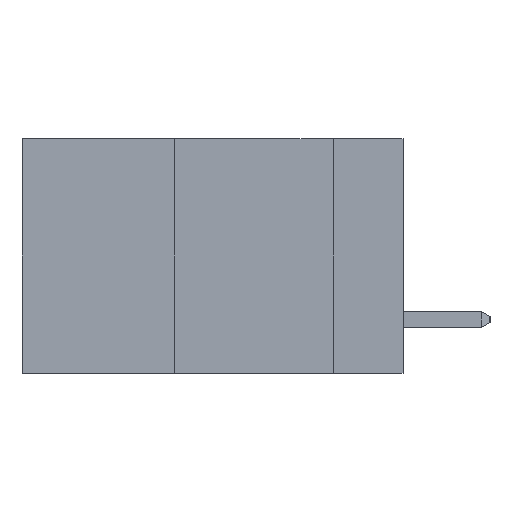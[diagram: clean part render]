
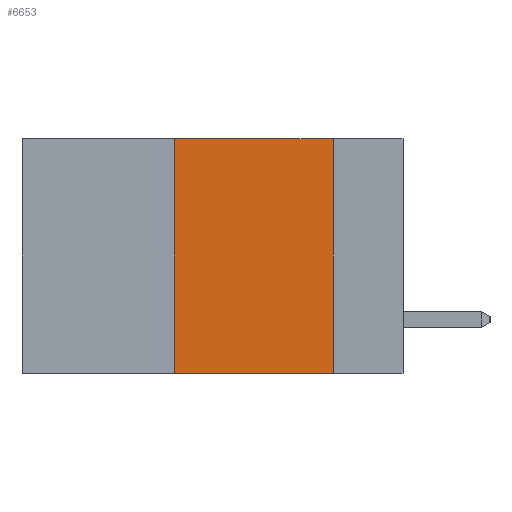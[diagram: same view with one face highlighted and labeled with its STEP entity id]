
A CAD part, left-side view. The second image highlights one B-rep face of the part: STEP entity #6653.
In plain terms, the highlighted planar face has unit normal (-1, 0, 0).
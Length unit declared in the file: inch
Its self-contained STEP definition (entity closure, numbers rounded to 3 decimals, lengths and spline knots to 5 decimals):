
#416 = DIRECTION ( 'NONE',  ( 0., 0., -1. ) ) ;
#819 = VECTOR ( 'NONE', #2534, 39.37008 ) ;
#1942 = EDGE_CURVE ( 'NONE', #12631, #17952, #3467, .T. ) ;
#2534 = DIRECTION ( 'NONE',  ( 0., -1., 0. ) ) ;
#2624 = CARTESIAN_POINT ( 'NONE',  ( 0., 0.11, -0.37 ) ) ;
#3456 = CARTESIAN_POINT ( 'NONE',  ( 0., 0.36, -0.37 ) ) ;
#3467 = LINE ( 'NONE', #4192, #819 ) ;
#3783 = VERTEX_POINT ( 'NONE', #3456 ) ;
#4192 = CARTESIAN_POINT ( 'NONE',  ( 0., 0.6, 0. ) ) ;
#5355 = DIRECTION ( 'NONE',  ( 0., 0., -1. ) ) ;
#6578 = EDGE_CURVE ( 'NONE', #3783, #12631, #14050, .T. ) ;
#6653 = ADVANCED_FACE ( 'NONE', ( #7644 ), #15486, .F. ) ;
#7644 = FACE_OUTER_BOUND ( 'NONE', #21055, .T. ) ;
#8362 = ORIENTED_EDGE ( 'NONE', *, *, #1942, .F. ) ;
#8482 = CARTESIAN_POINT ( 'NONE',  ( 0., 0.11, 0. ) ) ;
#8776 = CARTESIAN_POINT ( 'NONE',  ( 0., 0.6, 0. ) ) ;
#8978 = VERTEX_POINT ( 'NONE', #2624 ) ;
#10930 = AXIS2_PLACEMENT_3D ( 'NONE', #8776, #12283, #416 ) ;
#11363 = ORIENTED_EDGE ( 'NONE', *, *, #6578, .F. ) ;
#11662 = LINE ( 'NONE', #8482, #18514 ) ;
#11850 = EDGE_CURVE ( 'NONE', #3783, #8978, #19958, .T. ) ;
#12029 = ORIENTED_EDGE ( 'NONE', *, *, #11850, .T. ) ;
#12180 = CARTESIAN_POINT ( 'NONE',  ( 0., 0.36, 0. ) ) ;
#12283 = DIRECTION ( 'NONE',  ( 1., 0., 0. ) ) ;
#12631 = VERTEX_POINT ( 'NONE', #12180 ) ;
#13407 = ORIENTED_EDGE ( 'NONE', *, *, #21047, .F. ) ;
#14050 = LINE ( 'NONE', #20287, #16358 ) ;
#15025 = CARTESIAN_POINT ( 'NONE',  ( 0., 0.11, 0. ) ) ;
#15486 = PLANE ( 'NONE',  #10930 ) ;
#15491 = VECTOR ( 'NONE', #19817, 39.37008 ) ;
#16358 = VECTOR ( 'NONE', #20422, 39.37008 ) ;
#17952 = VERTEX_POINT ( 'NONE', #15025 ) ;
#18514 = VECTOR ( 'NONE', #5355, 39.37008 ) ;
#19672 = CARTESIAN_POINT ( 'NONE',  ( 0., 0.6, -0.37 ) ) ;
#19817 = DIRECTION ( 'NONE',  ( 0., -1., 0. ) ) ;
#19958 = LINE ( 'NONE', #19672, #15491 ) ;
#20287 = CARTESIAN_POINT ( 'NONE',  ( 0., 0.36, 0. ) ) ;
#20422 = DIRECTION ( 'NONE',  ( 0., 0., 1. ) ) ;
#21047 = EDGE_CURVE ( 'NONE', #17952, #8978, #11662, .T. ) ;
#21055 = EDGE_LOOP ( 'NONE', ( #13407, #8362, #11363, #12029 ) ) ;
